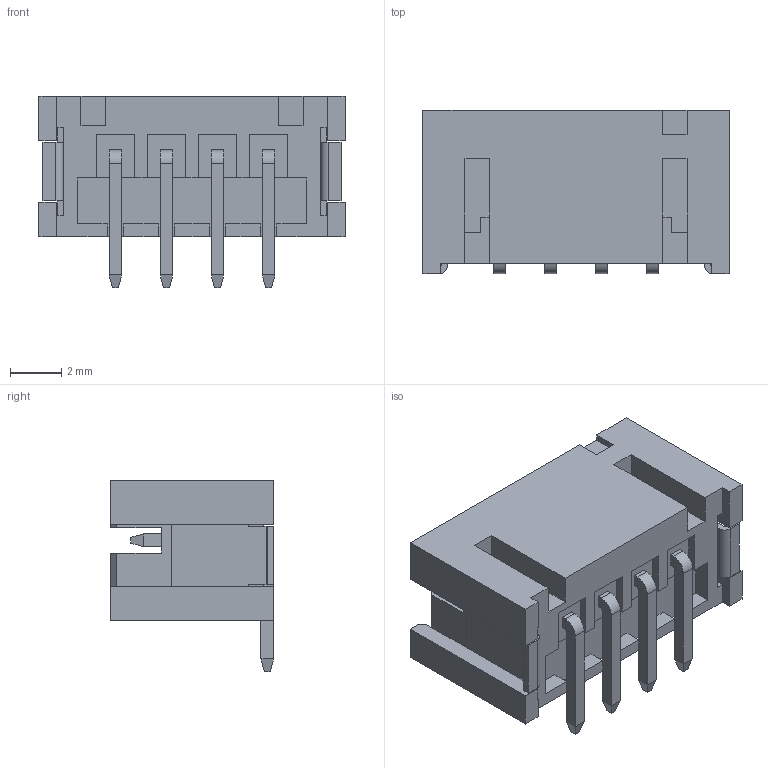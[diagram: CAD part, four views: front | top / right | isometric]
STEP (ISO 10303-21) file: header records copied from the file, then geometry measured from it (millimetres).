
FILE_DESCRIPTION (( 'STEP AP203' ), '1' );
FILE_NAME ('140-504-417-011.STEP', '2020-03-31T20:01:56', ( '' ), ( '' ), 'SwSTEP 2.0', 'SolidWorks 2016', '' );
FILE_SCHEMA (( 'CONFIG_CONTROL_DESIGN' ));
Length unit declared in the file: millimetre
Products named in the file (4): 140-504-417-011; V SMT Contact; V SMT Pad; V SMT Housing_504
Assembly tree (7 placements, depth 2):
  140-504-417-011
    V SMT Housing_504
    V SMT Contact  x4
    V SMT Pad  x2
Bounding box: 12 x 6.4 x 7.5 mm (x, y, z)
Volume: 196.7 mm3; surface area: 700.6 mm2
Topology: 7 solids, 7 shells, 252 faces, 652 edges, 410 vertices
Faces by surface type: plane 240, cylinder 12
Entity records: 5974 total; most frequent: CARTESIAN_POINT 980, ORIENTED_EDGE 968, DIRECTION 856, EDGE_CURVE 484, LINE 476, VECTOR 476, VERTEX_POINT 314, AXIS2_PLACEMENT_3D 190
